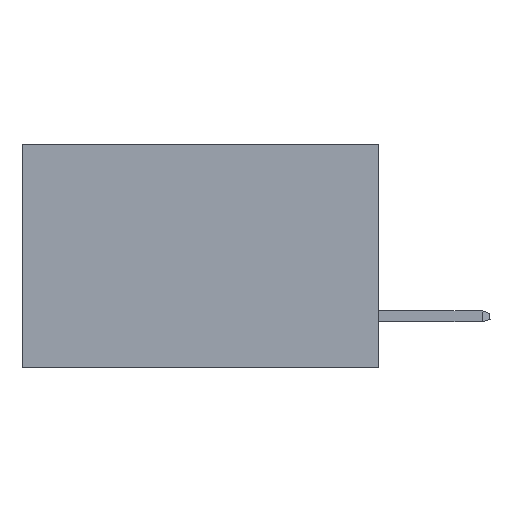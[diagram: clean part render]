
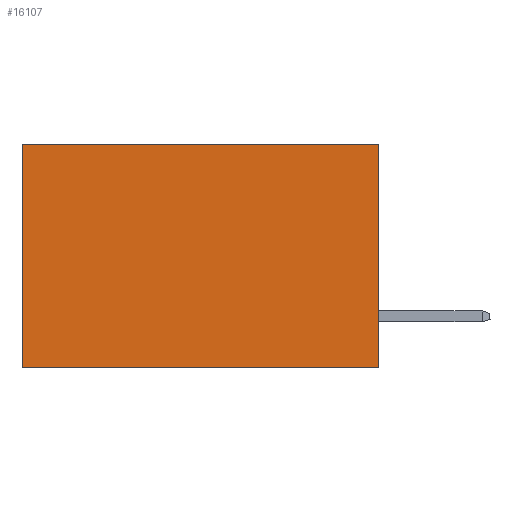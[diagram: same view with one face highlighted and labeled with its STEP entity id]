
A CAD part, left-side view. The second image highlights one B-rep face of the part: STEP entity #16107.
In plain terms, the highlighted planar face has unit normal (-1, 0, 0).
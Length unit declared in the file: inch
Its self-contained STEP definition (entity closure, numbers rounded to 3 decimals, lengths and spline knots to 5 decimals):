
#36 = CARTESIAN_POINT ( 'NONE',  ( 0.277, 0.59, -0.37 ) ) ;
#199 = VECTOR ( 'NONE', #11799, 39.37008 ) ;
#1020 = PLANE ( 'NONE',  #1956 ) ;
#1267 = CARTESIAN_POINT ( 'NONE',  ( 0.277, 0., 0. ) ) ;
#1273 = EDGE_CURVE ( 'NONE', #24220, #8756, #14698, .T. ) ;
#1956 = AXIS2_PLACEMENT_3D ( 'NONE', #16101, #4804, #17978 ) ;
#2413 = CARTESIAN_POINT ( 'NONE',  ( 0.277, 0., -0.37 ) ) ;
#4360 = LINE ( 'NONE', #12033, #23782 ) ;
#4804 = DIRECTION ( 'NONE',  ( 1., 0., 0. ) ) ;
#5503 = ORIENTED_EDGE ( 'NONE', *, *, #23296, .F. ) ;
#5803 = FACE_OUTER_BOUND ( 'NONE', #21379, .T. ) ;
#7306 = ORIENTED_EDGE ( 'NONE', *, *, #1273, .T. ) ;
#8756 = VERTEX_POINT ( 'NONE', #36 ) ;
#9507 = CARTESIAN_POINT ( 'NONE',  ( 0.277, 0.59, -0.37 ) ) ;
#9654 = ORIENTED_EDGE ( 'NONE', *, *, #10586, .F. ) ;
#10223 = VERTEX_POINT ( 'NONE', #1267 ) ;
#10586 = EDGE_CURVE ( 'NONE', #10223, #12195, #20205, .T. ) ;
#11634 = CARTESIAN_POINT ( 'NONE',  ( 0.277, 0., -0.37 ) ) ;
#11799 = DIRECTION ( 'NONE',  ( 0., 0., -1. ) ) ;
#12033 = CARTESIAN_POINT ( 'NONE',  ( 0.277, 0., -0.37 ) ) ;
#12195 = VERTEX_POINT ( 'NONE', #11634 ) ;
#12723 = VECTOR ( 'NONE', #18179, 39.37008 ) ;
#13931 = DIRECTION ( 'NONE',  ( 0., 1., 0. ) ) ;
#14698 = LINE ( 'NONE', #9507, #24087 ) ;
#14750 = CARTESIAN_POINT ( 'NONE',  ( 0.277, 0.59, 0. ) ) ;
#16101 = CARTESIAN_POINT ( 'NONE',  ( 0.277, 0., -0.37 ) ) ;
#16107 = ADVANCED_FACE ( 'NONE', ( #5803 ), #1020, .F. ) ;
#17978 = DIRECTION ( 'NONE',  ( 0., 0., -1. ) ) ;
#18179 = DIRECTION ( 'NONE',  ( 0., 1., 0. ) ) ;
#18986 = DIRECTION ( 'NONE',  ( 0., 0., -1. ) ) ;
#19001 = EDGE_CURVE ( 'NONE', #10223, #24220, #22735, .T. ) ;
#20205 = LINE ( 'NONE', #2413, #199 ) ;
#21379 = EDGE_LOOP ( 'NONE', ( #7306, #5503, #9654, #24316 ) ) ;
#22735 = LINE ( 'NONE', #23772, #12723 ) ;
#23296 = EDGE_CURVE ( 'NONE', #12195, #8756, #4360, .T. ) ;
#23772 = CARTESIAN_POINT ( 'NONE',  ( 0.277, 0., 0. ) ) ;
#23782 = VECTOR ( 'NONE', #13931, 39.37008 ) ;
#24087 = VECTOR ( 'NONE', #18986, 39.37008 ) ;
#24220 = VERTEX_POINT ( 'NONE', #14750 ) ;
#24316 = ORIENTED_EDGE ( 'NONE', *, *, #19001, .T. ) ;
